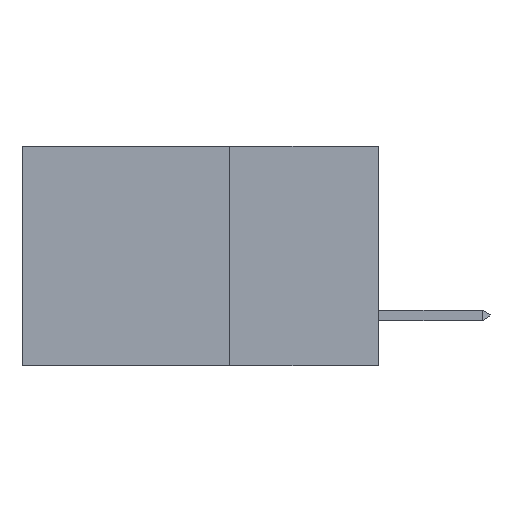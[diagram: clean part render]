
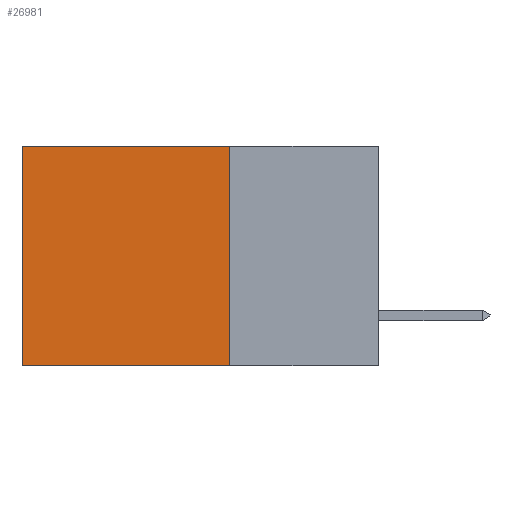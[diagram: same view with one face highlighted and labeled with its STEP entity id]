
A CAD part, left-side view. The second image highlights one B-rep face of the part: STEP entity #26981.
In plain terms, the highlighted planar face has unit normal (-1, 0, 0).
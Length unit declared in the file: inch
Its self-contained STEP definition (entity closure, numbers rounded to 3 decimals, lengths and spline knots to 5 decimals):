
#694 = CARTESIAN_POINT ( 'NONE',  ( 0.298, 0.25, -0.37 ) ) ;
#1333 = CARTESIAN_POINT ( 'NONE',  ( 0.298, 0.25, 0. ) ) ;
#2215 = EDGE_CURVE ( 'NONE', #6775, #13683, #9174, .T. ) ;
#2524 = DIRECTION ( 'NONE',  ( 0., 0., -1. ) ) ;
#3419 = VECTOR ( 'NONE', #2524, 39.37008 ) ;
#3640 = VECTOR ( 'NONE', #7395, 39.37008 ) ;
#4014 = EDGE_CURVE ( 'NONE', #12453, #12590, #13901, .T. ) ;
#4962 = CARTESIAN_POINT ( 'NONE',  ( 0.298, 0.25, 0. ) ) ;
#5481 = CARTESIAN_POINT ( 'NONE',  ( 0.298, 0.25, 0. ) ) ;
#6431 = VECTOR ( 'NONE', #15169, 39.37008 ) ;
#6775 = VERTEX_POINT ( 'NONE', #5481 ) ;
#6802 = ORIENTED_EDGE ( 'NONE', *, *, #4014, .F. ) ;
#7116 = CARTESIAN_POINT ( 'NONE',  ( 0.298, 0.25, 0. ) ) ;
#7217 = FACE_OUTER_BOUND ( 'NONE', #26380, .T. ) ;
#7368 = PLANE ( 'NONE',  #13354 ) ;
#7395 = DIRECTION ( 'NONE',  ( 0., 1., 0. ) ) ;
#7993 = VECTOR ( 'NONE', #16161, 39.37008 ) ;
#9174 = LINE ( 'NONE', #7116, #3640 ) ;
#10918 = CARTESIAN_POINT ( 'NONE',  ( 0.298, 0.6, 0. ) ) ;
#11916 = DIRECTION ( 'NONE',  ( 0., 0., -1. ) ) ;
#11996 = LINE ( 'NONE', #4962, #6431 ) ;
#12285 = EDGE_CURVE ( 'NONE', #13683, #12590, #16774, .T. ) ;
#12453 = VERTEX_POINT ( 'NONE', #694 ) ;
#12590 = VERTEX_POINT ( 'NONE', #22012 ) ;
#13354 = AXIS2_PLACEMENT_3D ( 'NONE', #1333, #17849, #11916 ) ;
#13683 = VERTEX_POINT ( 'NONE', #26516 ) ;
#13901 = LINE ( 'NONE', #26530, #7993 ) ;
#15169 = DIRECTION ( 'NONE',  ( 0., 0., -1. ) ) ;
#15908 = EDGE_CURVE ( 'NONE', #6775, #12453, #11996, .T. ) ;
#16161 = DIRECTION ( 'NONE',  ( 0., 1., 0. ) ) ;
#16774 = LINE ( 'NONE', #10918, #3419 ) ;
#17849 = DIRECTION ( 'NONE',  ( 1., 0., 0. ) ) ;
#18595 = ORIENTED_EDGE ( 'NONE', *, *, #2215, .T. ) ;
#19887 = ORIENTED_EDGE ( 'NONE', *, *, #12285, .T. ) ;
#22012 = CARTESIAN_POINT ( 'NONE',  ( 0.298, 0.6, -0.37 ) ) ;
#23332 = ORIENTED_EDGE ( 'NONE', *, *, #15908, .F. ) ;
#26380 = EDGE_LOOP ( 'NONE', ( #19887, #6802, #23332, #18595 ) ) ;
#26516 = CARTESIAN_POINT ( 'NONE',  ( 0.298, 0.6, 0. ) ) ;
#26530 = CARTESIAN_POINT ( 'NONE',  ( 0.298, 0.25, -0.37 ) ) ;
#26981 = ADVANCED_FACE ( 'NONE', ( #7217 ), #7368, .F. ) ;
